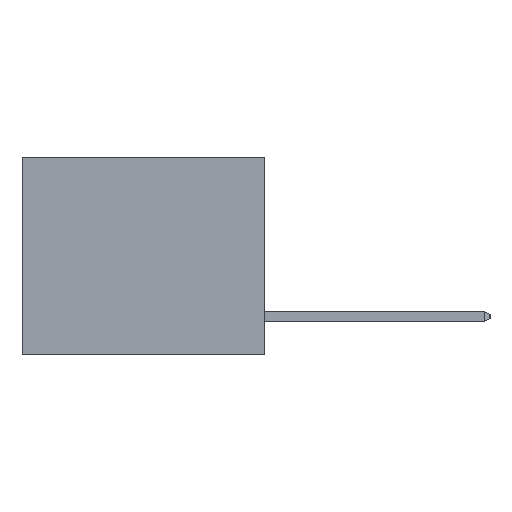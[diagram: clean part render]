
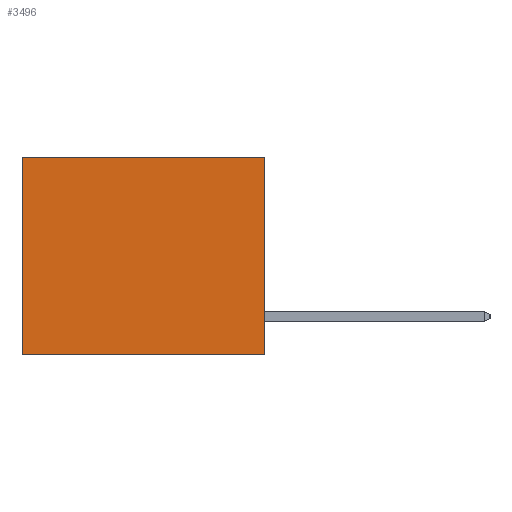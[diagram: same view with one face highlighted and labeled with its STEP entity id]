
A CAD part, left-side view. The second image highlights one B-rep face of the part: STEP entity #3496.
In plain terms, the highlighted planar face has unit normal (-1, 0, 0).
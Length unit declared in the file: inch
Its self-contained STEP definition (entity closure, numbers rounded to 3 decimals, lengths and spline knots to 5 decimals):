
#42 = VERTEX_POINT ( 'NONE', #665 ) ;
#654 = DIRECTION ( 'NONE',  ( 0., 0., -1. ) ) ;
#665 = CARTESIAN_POINT ( 'NONE',  ( 0.3165, 0.6, -0.49 ) ) ;
#997 = ORIENTED_EDGE ( 'NONE', *, *, #25651, .T. ) ;
#2272 = CARTESIAN_POINT ( 'NONE',  ( 0.3165, 0., 0. ) ) ;
#3496 = ADVANCED_FACE ( 'NONE', ( #20901 ), #21288, .F. ) ;
#3705 = EDGE_CURVE ( 'NONE', #15318, #14730, #23426, .T. ) ;
#4274 = VECTOR ( 'NONE', #4731, 39.37008 ) ;
#4731 = DIRECTION ( 'NONE',  ( 0., 0., -1. ) ) ;
#4850 = CARTESIAN_POINT ( 'NONE',  ( 0.3165, 0., -0.49 ) ) ;
#5692 = ORIENTED_EDGE ( 'NONE', *, *, #7959, .T. ) ;
#7083 = DIRECTION ( 'NONE',  ( 0., 1., 0. ) ) ;
#7959 = EDGE_CURVE ( 'NONE', #15318, #22032, #13593, .T. ) ;
#9069 = CARTESIAN_POINT ( 'NONE',  ( 0.3165, 0., -0.49 ) ) ;
#9292 = EDGE_LOOP ( 'NONE', ( #997, #14418, #18628, #5692 ) ) ;
#11116 = DIRECTION ( 'NONE',  ( 0., 0., -1. ) ) ;
#11456 = AXIS2_PLACEMENT_3D ( 'NONE', #9069, #23318, #11116 ) ;
#12531 = CARTESIAN_POINT ( 'NONE',  ( 0.3165, 0., -0.49 ) ) ;
#12864 = CARTESIAN_POINT ( 'NONE',  ( 0.3165, 0.6, -0.49 ) ) ;
#13192 = CARTESIAN_POINT ( 'NONE',  ( 0.3165, 0.6, 0. ) ) ;
#13593 = LINE ( 'NONE', #24959, #26268 ) ;
#14418 = ORIENTED_EDGE ( 'NONE', *, *, #19771, .F. ) ;
#14730 = VERTEX_POINT ( 'NONE', #12531 ) ;
#15150 = CARTESIAN_POINT ( 'NONE',  ( 0.3165, 0., -0.49 ) ) ;
#15318 = VERTEX_POINT ( 'NONE', #2272 ) ;
#18006 = LINE ( 'NONE', #12864, #4274 ) ;
#18335 = LINE ( 'NONE', #15150, #20244 ) ;
#18628 = ORIENTED_EDGE ( 'NONE', *, *, #3705, .F. ) ;
#19625 = VECTOR ( 'NONE', #654, 39.37008 ) ;
#19771 = EDGE_CURVE ( 'NONE', #14730, #42, #18335, .T. ) ;
#20244 = VECTOR ( 'NONE', #25500, 39.37008 ) ;
#20901 = FACE_OUTER_BOUND ( 'NONE', #9292, .T. ) ;
#21288 = PLANE ( 'NONE',  #11456 ) ;
#22032 = VERTEX_POINT ( 'NONE', #13192 ) ;
#23318 = DIRECTION ( 'NONE',  ( 1., 0., 0. ) ) ;
#23426 = LINE ( 'NONE', #4850, #19625 ) ;
#24959 = CARTESIAN_POINT ( 'NONE',  ( 0.3165, 0., 0. ) ) ;
#25500 = DIRECTION ( 'NONE',  ( 0., 1., 0. ) ) ;
#25651 = EDGE_CURVE ( 'NONE', #22032, #42, #18006, .T. ) ;
#26268 = VECTOR ( 'NONE', #7083, 39.37008 ) ;
